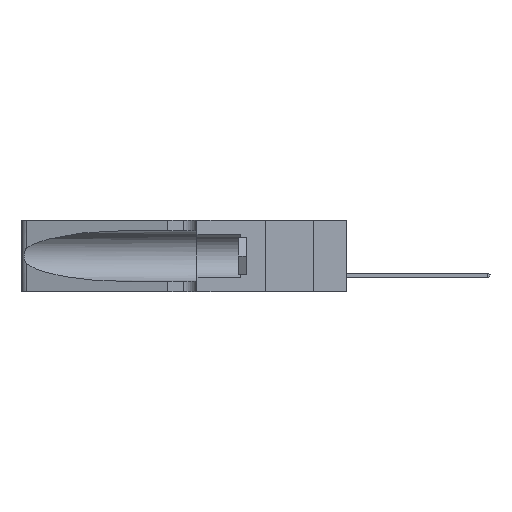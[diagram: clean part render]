
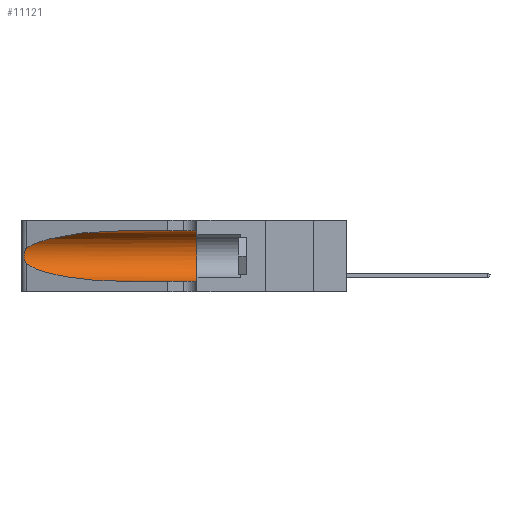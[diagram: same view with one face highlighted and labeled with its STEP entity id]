
A CAD part, left-side view. The second image highlights one B-rep face of the part: STEP entity #11121.
In plain terms, the highlighted cylindrical face has radius 3.308 mm (diameter 6.617 mm), a partial arc.
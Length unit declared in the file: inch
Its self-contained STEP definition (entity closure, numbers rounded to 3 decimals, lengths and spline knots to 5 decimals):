
#1895 = CARTESIAN_POINT ( 'NONE',  ( 0.25789, 1.23486, 0.15765 ) ) ;
#1998 = EDGE_CURVE ( 'NONE', #3684, #15210, #13425, .T. ) ;
#2077 = CARTESIAN_POINT ( 'NONE',  ( 0.25856, 1.23593, 0.16098 ) ) ;
#2082 = CARTESIAN_POINT ( 'NONE',  ( 0.1305, 0.35, 0.05475 ) ) ;
#3209 = DIRECTION ( 'NONE',  ( 0., -1., 0. ) ) ;
#3345 = CARTESIAN_POINT ( 'NONE',  ( 0.25487, 1.22718, 0.14631 ) ) ;
#3417 = LINE ( 'NONE', #6457, #29335 ) ;
#3684 = VERTEX_POINT ( 'NONE', #11567 ) ;
#4214 = AXIS2_PLACEMENT_3D ( 'NONE', #21393, #19209, #5573 ) ;
#5573 = DIRECTION ( 'NONE',  ( 0., 0., 1. ) ) ;
#5600 = EDGE_CURVE ( 'NONE', #15210, #25612, #27266, .T. ) ;
#6457 = CARTESIAN_POINT ( 'NONE',  ( 0.1305, 1.61858, 0.31525 ) ) ;
#6616 = EDGE_CURVE ( 'NONE', #25612, #9507, #9667, .T. ) ;
#7290 = CARTESIAN_POINT ( 'NONE',  ( 0.1305, 0.72297, 0.05475 ) ) ;
#7789 = ORIENTED_EDGE ( 'NONE', *, *, #5600, .T. ) ;
#8333 = VERTEX_POINT ( 'NONE', #27509 ) ;
#8724 = CARTESIAN_POINT ( 'NONE',  ( 0.2373, 1.15595, 0.28018 ) ) ;
#8889 = CARTESIAN_POINT ( 'NONE',  ( 0.25487, 1.22718, 0.22369 ) ) ;
#8987 = CARTESIAN_POINT ( 'NONE',  ( 0.25555, 1.22993, 0.14849 ) ) ;
#9443 = DIRECTION ( 'NONE',  ( 0., -1., 0. ) ) ;
#9507 = VERTEX_POINT ( 'NONE', #7290 ) ;
#9667 =( BOUNDED_CURVE ( )  B_SPLINE_CURVE ( 3, ( #14962, #19515, #11551, #15810 ),
 .UNSPECIFIED., .F., .F. ) 
 B_SPLINE_CURVE_WITH_KNOTS ( ( 4, 4 ),
 ( 3.44316, 4.71239 ),
 .UNSPECIFIED. ) 
 CURVE ( )  GEOMETRIC_REPRESENTATION_ITEM ( )  RATIONAL_B_SPLINE_CURVE ( ( 1., 0.87, 0.87, 1. ) ) 
 REPRESENTATION_ITEM ( '' )  );
#10746 = FACE_OUTER_BOUND ( 'NONE', #29327, .T. ) ;
#11121 = ADVANCED_FACE ( 'NONE', ( #10746 ), #24896, .F. ) ;
#11551 = CARTESIAN_POINT ( 'NONE',  ( 0.18966, 0.96281, 0.05475 ) ) ;
#11567 = CARTESIAN_POINT ( 'NONE',  ( 0.1305, 0.72297, 0.31525 ) ) ;
#12345 = CARTESIAN_POINT ( 'NONE',  ( 0.1305, 1.61858, 0.05475 ) ) ;
#12832 = CARTESIAN_POINT ( 'NONE',  ( 0.1305, 1.61858, 0.185 ) ) ;
#13409 = ORIENTED_EDGE ( 'NONE', *, *, #1998, .T. ) ;
#13425 =( BOUNDED_CURVE ( )  B_SPLINE_CURVE ( 3, ( #24484, #17750, #8724, #24577 ),
 .UNSPECIFIED., .F., .F. ) 
 B_SPLINE_CURVE_WITH_KNOTS ( ( 4, 4 ),
 ( 1.5708, 2.84003 ),
 .UNSPECIFIED. ) 
 CURVE ( )  GEOMETRIC_REPRESENTATION_ITEM ( )  RATIONAL_B_SPLINE_CURVE ( ( 1., 0.87, 0.87, 1. ) ) 
 REPRESENTATION_ITEM ( '' )  );
#13495 = EDGE_CURVE ( 'NONE', #8333, #25366, #23236, .T. ) ;
#13571 = CARTESIAN_POINT ( 'NONE',  ( 0.25639, 1.23186, 0.15144 ) ) ;
#14863 = ORIENTED_EDGE ( 'NONE', *, *, #17231, .F. ) ;
#14962 = CARTESIAN_POINT ( 'NONE',  ( 0.25487, 1.22718, 0.14631 ) ) ;
#15210 = VERTEX_POINT ( 'NONE', #21570 ) ;
#15545 = CARTESIAN_POINT ( 'NONE',  ( 0.25854, 1.2359, 0.20912 ) ) ;
#15741 = CARTESIAN_POINT ( 'NONE',  ( 0.26017, 1.23833, 0.17102 ) ) ;
#15810 = CARTESIAN_POINT ( 'NONE',  ( 0.1305, 0.72297, 0.05475 ) ) ;
#17231 = EDGE_CURVE ( 'NONE', #3684, #8333, #3417, .T. ) ;
#17650 = DIRECTION ( 'NONE',  ( 0., 0., -1. ) ) ;
#17750 = CARTESIAN_POINT ( 'NONE',  ( 0.18966, 0.96281, 0.31525 ) ) ;
#19209 = DIRECTION ( 'NONE',  ( 0., 1., 0. ) ) ;
#19515 = CARTESIAN_POINT ( 'NONE',  ( 0.2373, 1.15595, 0.08982 ) ) ;
#21393 = CARTESIAN_POINT ( 'NONE',  ( 0.1305, 0.35, 0.185 ) ) ;
#21570 = CARTESIAN_POINT ( 'NONE',  ( 0.25487, 1.22718, 0.22369 ) ) ;
#22569 = CARTESIAN_POINT ( 'NONE',  ( 0.26075, 1.23896, 0.178 ) ) ;
#22601 = DIRECTION ( 'NONE',  ( 0., -1., 0. ) ) ;
#22720 = VECTOR ( 'NONE', #3209, 39.37008 ) ;
#23236 = CIRCLE ( 'NONE', #4214, 0.13025 ) ;
#24444 = EDGE_CURVE ( 'NONE', #9507, #25366, #26574, .T. ) ;
#24484 = CARTESIAN_POINT ( 'NONE',  ( 0.1305, 0.72297, 0.31525 ) ) ;
#24577 = CARTESIAN_POINT ( 'NONE',  ( 0.25487, 1.22718, 0.22369 ) ) ;
#24731 = CARTESIAN_POINT ( 'NONE',  ( 0.25639, 1.23184, 0.21858 ) ) ;
#24828 = CARTESIAN_POINT ( 'NONE',  ( 0.25787, 1.23484, 0.2124 ) ) ;
#24896 = CYLINDRICAL_SURFACE ( 'NONE', #26434, 0.13025 ) ;
#25100 = ORIENTED_EDGE ( 'NONE', *, *, #6616, .T. ) ;
#25366 = VERTEX_POINT ( 'NONE', #2082 ) ;
#25612 = VERTEX_POINT ( 'NONE', #3345 ) ;
#26434 = AXIS2_PLACEMENT_3D ( 'NONE', #12832, #22601, #17650 ) ;
#26574 = LINE ( 'NONE', #12345, #22720 ) ;
#26873 = ORIENTED_EDGE ( 'NONE', *, *, #13495, .F. ) ;
#26982 = CARTESIAN_POINT ( 'NONE',  ( 0.26018, 1.23835, 0.19895 ) ) ;
#27074 = CARTESIAN_POINT ( 'NONE',  ( 0.25555, 1.22994, 0.2215 ) ) ;
#27266 = B_SPLINE_CURVE_WITH_KNOTS ( 'NONE', 3,
 ( #8889, #27074, #24731, #24828, #15545, #26982, #29241, #22569, #15741, #2077, #1895, #13571, #8987, #29339 ),
 .UNSPECIFIED., .F., .F.,
 ( 4, 2, 2, 2, 2, 2, 4 ),
 ( 0., 0.00027, 0.00053, 0.00107, 0.0016, 0.00187, 0.00214 ),
 .UNSPECIFIED. ) ;
#27509 = CARTESIAN_POINT ( 'NONE',  ( 0.1305, 0.35, 0.31525 ) ) ;
#28380 = ORIENTED_EDGE ( 'NONE', *, *, #24444, .T. ) ;
#29241 = CARTESIAN_POINT ( 'NONE',  ( 0.26075, 1.23896, 0.19203 ) ) ;
#29327 = EDGE_LOOP ( 'NONE', ( #13409, #7789, #25100, #28380, #26873, #14863 ) ) ;
#29335 = VECTOR ( 'NONE', #9443, 39.37008 ) ;
#29339 = CARTESIAN_POINT ( 'NONE',  ( 0.25487, 1.22718, 0.14631 ) ) ;
